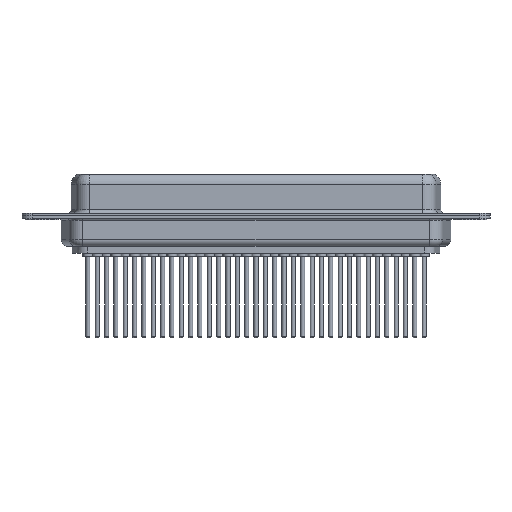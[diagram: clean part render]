
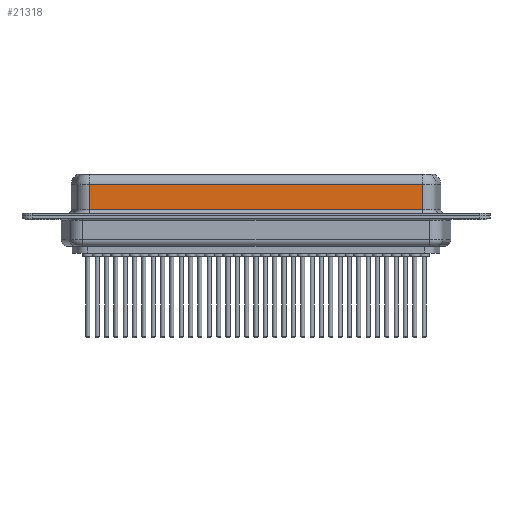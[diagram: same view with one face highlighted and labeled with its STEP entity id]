
A CAD part, front view. The second image highlights one B-rep face of the part: STEP entity #21318.
In plain terms, the highlighted planar face has unit normal (0, -1, 0).
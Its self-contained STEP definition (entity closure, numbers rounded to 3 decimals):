
#62 = CARTESIAN_POINT ( 'NONE',  ( 7.038, -3.95, 0.9 ) ) ;
#378 = VERTEX_POINT ( 'NONE', #22550 ) ;
#547 = LINE ( 'NONE', #2313, #13457 ) ;
#585 = AXIS2_PLACEMENT_3D ( 'NONE', #17003, #15273, #7846 ) ;
#807 = DIRECTION ( 'NONE',  ( -1., 0., 0. ) ) ;
#2089 = VERTEX_POINT ( 'NONE', #22709 ) ;
#2313 = CARTESIAN_POINT ( 'NONE',  ( 56.462, -3.95, 4.65 ) ) ;
#2528 = LINE ( 'NONE', #10149, #16517 ) ;
#2689 = LINE ( 'NONE', #14602, #18617 ) ;
#3566 = CARTESIAN_POINT ( 'NONE',  ( 56.462, -3.95, 0.9 ) ) ;
#4820 = EDGE_CURVE ( 'NONE', #2089, #12008, #2528, .T. ) ;
#5584 = ORIENTED_EDGE ( 'NONE', *, *, #17882, .T. ) ;
#7846 = DIRECTION ( 'NONE',  ( -1., 0., 0. ) ) ;
#8294 = DIRECTION ( 'NONE',  ( 0., 0., -1. ) ) ;
#9012 = EDGE_LOOP ( 'NONE', ( #12878, #11272, #5584, #22713 ) ) ;
#10149 = CARTESIAN_POINT ( 'NONE',  ( 56.462, -3.95, 6.4 ) ) ;
#11272 = ORIENTED_EDGE ( 'NONE', *, *, #23320, .T. ) ;
#12008 = VERTEX_POINT ( 'NONE', #3566 ) ;
#12175 = LINE ( 'NONE', #23945, #21749 ) ;
#12878 = ORIENTED_EDGE ( 'NONE', *, *, #4820, .F. ) ;
#13457 = VECTOR ( 'NONE', #807, 1000. ) ;
#14471 = DIRECTION ( 'NONE',  ( 1., 0., 0. ) ) ;
#14602 = CARTESIAN_POINT ( 'NONE',  ( 7.038, -3.95, 6.4 ) ) ;
#15273 = DIRECTION ( 'NONE',  ( 0., 1., 0. ) ) ;
#16517 = VECTOR ( 'NONE', #8294, 1000. ) ;
#17003 = CARTESIAN_POINT ( 'NONE',  ( 56.462, -3.95, 6.4 ) ) ;
#17882 = EDGE_CURVE ( 'NONE', #378, #20461, #2689, .T. ) ;
#18617 = VECTOR ( 'NONE', #24079, 1000. ) ;
#19248 = FACE_OUTER_BOUND ( 'NONE', #9012, .T. ) ;
#20461 = VERTEX_POINT ( 'NONE', #62 ) ;
#20668 = EDGE_CURVE ( 'NONE', #20461, #12008, #12175, .T. ) ;
#21318 = ADVANCED_FACE ( 'NONE', ( #19248 ), #24504, .F. ) ;
#21749 = VECTOR ( 'NONE', #14471, 1000. ) ;
#22550 = CARTESIAN_POINT ( 'NONE',  ( 7.038, -3.95, 4.65 ) ) ;
#22709 = CARTESIAN_POINT ( 'NONE',  ( 56.462, -3.95, 4.65 ) ) ;
#22713 = ORIENTED_EDGE ( 'NONE', *, *, #20668, .T. ) ;
#23320 = EDGE_CURVE ( 'NONE', #2089, #378, #547, .T. ) ;
#23945 = CARTESIAN_POINT ( 'NONE',  ( 56.462, -3.95, 0.9 ) ) ;
#24079 = DIRECTION ( 'NONE',  ( 0., 0., -1. ) ) ;
#24504 = PLANE ( 'NONE',  #585 ) ;
